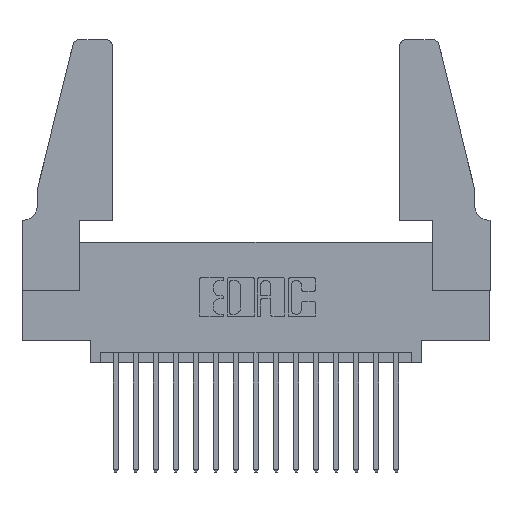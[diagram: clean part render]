
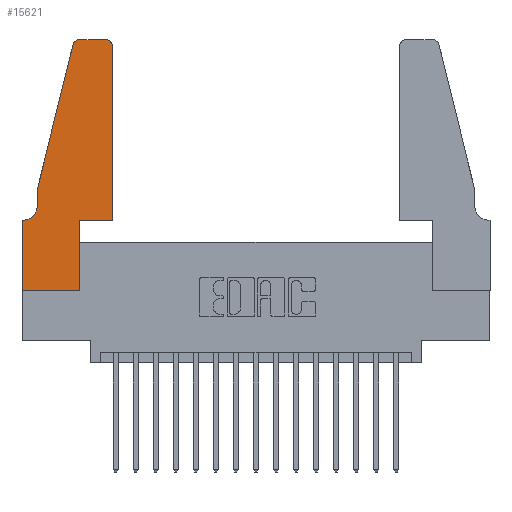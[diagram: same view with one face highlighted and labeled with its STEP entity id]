
A CAD part, top view. The second image highlights one B-rep face of the part: STEP entity #15621.
In plain terms, the highlighted planar face has unit normal (0, 0, 1).
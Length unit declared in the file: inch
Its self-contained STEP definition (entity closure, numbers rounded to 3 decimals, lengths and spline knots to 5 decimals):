
#3 = ORIENTED_EDGE ( 'NONE', *, *, #2744, .T. ) ;
#227 = EDGE_CURVE ( 'NONE', #11951, #13498, #530, .T. ) ;
#426 = CARTESIAN_POINT ( 'NONE',  ( 0.4505, 0.35, 0.37 ) ) ;
#530 = CIRCLE ( 'NONE', #17356, 0.03 ) ;
#564 = ORIENTED_EDGE ( 'NONE', *, *, #10258, .T. ) ;
#593 = CARTESIAN_POINT ( 'NONE',  ( 0.25487, 1.22718, 0.37 ) ) ;
#733 = CARTESIAN_POINT ( 'NONE',  ( 0.284, 1.22, 0.37 ) ) ;
#1566 = LINE ( 'NONE', #4669, #15255 ) ;
#1813 = LINE ( 'NONE', #7935, #13168 ) ;
#1875 = DIRECTION ( 'NONE',  ( 1., 0., 0. ) ) ;
#1921 = DIRECTION ( 'NONE',  ( 0., 0., 1. ) ) ;
#2294 = LINE ( 'NONE', #15361, #9162 ) ;
#2454 = DIRECTION ( 'NONE',  ( 0., 0., 1. ) ) ;
#2741 = ORIENTED_EDGE ( 'NONE', *, *, #15988, .T. ) ;
#2744 = EDGE_CURVE ( 'NONE', #3467, #5222, #1566, .T. ) ;
#2806 = CARTESIAN_POINT ( 'NONE',  ( 0.284, 1.25, 0.37 ) ) ;
#3303 = DIRECTION ( 'NONE',  ( 1., 0., 0. ) ) ;
#3320 = DIRECTION ( 'NONE',  ( 0., 0., 1. ) ) ;
#3467 = VERTEX_POINT ( 'NONE', #4648 ) ;
#3712 = EDGE_CURVE ( 'NONE', #12229, #3467, #1813, .T. ) ;
#4157 = DIRECTION ( 'NONE',  ( -0.239, -0.971, 0. ) ) ;
#4330 = VERTEX_POINT ( 'NONE', #14468 ) ;
#4384 = VECTOR ( 'NONE', #11359, 39.37008 ) ;
#4648 = CARTESIAN_POINT ( 'NONE',  ( 0., 0.35, 0.37 ) ) ;
#4669 = CARTESIAN_POINT ( 'NONE',  ( 0., 0., 0.37 ) ) ;
#4697 = EDGE_CURVE ( 'NONE', #10967, #6878, #7369, .T. ) ;
#5222 = VERTEX_POINT ( 'NONE', #8306 ) ;
#5450 = CARTESIAN_POINT ( 'NONE',  ( 0.0055, 0.42, 0.37 ) ) ;
#5584 = LINE ( 'NONE', #16413, #12421 ) ;
#5841 = DIRECTION ( 'NONE',  ( -1., 0., 0. ) ) ;
#5946 = EDGE_LOOP ( 'NONE', ( #8608, #14848, #11247, #11374, #2741, #7459, #3, #564, #16889, #15069, #6628, #9710 ) ) ;
#6025 = LINE ( 'NONE', #16396, #16035 ) ;
#6541 = CARTESIAN_POINT ( 'NONE',  ( 0.2865, 0., 0.37 ) ) ;
#6548 = AXIS2_PLACEMENT_3D ( 'NONE', #10142, #1921, #11499 ) ;
#6549 = VERTEX_POINT ( 'NONE', #14951 ) ;
#6628 = ORIENTED_EDGE ( 'NONE', *, *, #9845, .T. ) ;
#6826 = DIRECTION ( 'NONE',  ( -1., 0., 0. ) ) ;
#6878 = VERTEX_POINT ( 'NONE', #15640 ) ;
#7225 = CARTESIAN_POINT ( 'NONE',  ( 0.0755, 0.5, 0.37 ) ) ;
#7266 = EDGE_CURVE ( 'NONE', #13498, #10967, #5584, .T. ) ;
#7333 = FACE_OUTER_BOUND ( 'NONE', #5946, .T. ) ;
#7369 = LINE ( 'NONE', #10011, #4384 ) ;
#7459 = ORIENTED_EDGE ( 'NONE', *, *, #3712, .T. ) ;
#7738 = AXIS2_PLACEMENT_3D ( 'NONE', #11516, #3320, #12883 ) ;
#7935 = CARTESIAN_POINT ( 'NONE',  ( 0.0755, 0.35, 0.37 ) ) ;
#8149 = CIRCLE ( 'NONE', #7738, 0.03 ) ;
#8169 = VECTOR ( 'NONE', #15544, 39.37008 ) ;
#8306 = CARTESIAN_POINT ( 'NONE',  ( 0., 0., 0.37 ) ) ;
#8599 = LINE ( 'NONE', #14199, #8169 ) ;
#8608 = ORIENTED_EDGE ( 'NONE', *, *, #9064, .T. ) ;
#9064 = EDGE_CURVE ( 'NONE', #16120, #11951, #2294, .T. ) ;
#9162 = VECTOR ( 'NONE', #5841, 39.37008 ) ;
#9217 = AXIS2_PLACEMENT_3D ( 'NONE', #5450, #14985, #6826 ) ;
#9274 = LINE ( 'NONE', #15568, #12462 ) ;
#9710 = ORIENTED_EDGE ( 'NONE', *, *, #11013, .T. ) ;
#9845 = EDGE_CURVE ( 'NONE', #6549, #11124, #9274, .T. ) ;
#10011 = CARTESIAN_POINT ( 'NONE',  ( 0.0755, 0.5, 0.37 ) ) ;
#10142 = CARTESIAN_POINT ( 'NONE',  ( 0., 0.35, 0.37 ) ) ;
#10258 = EDGE_CURVE ( 'NONE', #5222, #17275, #6025, .T. ) ;
#10285 = LINE ( 'NONE', #426, #16645 ) ;
#10512 = EDGE_CURVE ( 'NONE', #17275, #4330, #8599, .T. ) ;
#10967 = VERTEX_POINT ( 'NONE', #7225 ) ;
#11013 = EDGE_CURVE ( 'NONE', #11124, #16120, #8149, .T. ) ;
#11124 = VERTEX_POINT ( 'NONE', #17143 ) ;
#11247 = ORIENTED_EDGE ( 'NONE', *, *, #7266, .T. ) ;
#11359 = DIRECTION ( 'NONE',  ( 0., -1., 0. ) ) ;
#11374 = ORIENTED_EDGE ( 'NONE', *, *, #4697, .T. ) ;
#11499 = DIRECTION ( 'NONE',  ( 1., 0., 0. ) ) ;
#11516 = CARTESIAN_POINT ( 'NONE',  ( 0.4205, 1.22, 0.37 ) ) ;
#11594 = CARTESIAN_POINT ( 'NONE',  ( 0.0055, 0.35, 0.37 ) ) ;
#11951 = VERTEX_POINT ( 'NONE', #2806 ) ;
#12229 = VERTEX_POINT ( 'NONE', #11594 ) ;
#12421 = VECTOR ( 'NONE', #4157, 39.37008 ) ;
#12462 = VECTOR ( 'NONE', #16941, 39.37008 ) ;
#12559 = CARTESIAN_POINT ( 'NONE',  ( 0.4205, 1.25, 0.37 ) ) ;
#12655 = CIRCLE ( 'NONE', #9217, 0.07 ) ;
#12883 = DIRECTION ( 'NONE',  ( 1., 0., 0. ) ) ;
#13168 = VECTOR ( 'NONE', #16006, 39.37008 ) ;
#13498 = VERTEX_POINT ( 'NONE', #593 ) ;
#14199 = CARTESIAN_POINT ( 'NONE',  ( 0.2865, 0.35, 0.37 ) ) ;
#14209 = DIRECTION ( 'NONE',  ( 0., -1., 0. ) ) ;
#14468 = CARTESIAN_POINT ( 'NONE',  ( 0.2865, 0.35, 0.37 ) ) ;
#14848 = ORIENTED_EDGE ( 'NONE', *, *, #227, .T. ) ;
#14951 = CARTESIAN_POINT ( 'NONE',  ( 0.4505, 0.35, 0.37 ) ) ;
#14985 = DIRECTION ( 'NONE',  ( 0., 0., -1. ) ) ;
#15035 = DIRECTION ( 'NONE',  ( 1., 0., 0. ) ) ;
#15069 = ORIENTED_EDGE ( 'NONE', *, *, #16872, .T. ) ;
#15255 = VECTOR ( 'NONE', #14209, 39.37008 ) ;
#15361 = CARTESIAN_POINT ( 'NONE',  ( 0.2605, 1.25, 0.37 ) ) ;
#15544 = DIRECTION ( 'NONE',  ( 0., 1., 0. ) ) ;
#15568 = CARTESIAN_POINT ( 'NONE',  ( 0.4505, 0.35, 0.37 ) ) ;
#15621 = ADVANCED_FACE ( 'NONE', ( #7333 ), #16887, .T. ) ;
#15640 = CARTESIAN_POINT ( 'NONE',  ( 0.0755, 0.42, 0.37 ) ) ;
#15988 = EDGE_CURVE ( 'NONE', #6878, #12229, #12655, .T. ) ;
#16006 = DIRECTION ( 'NONE',  ( -1., 0., 0. ) ) ;
#16035 = VECTOR ( 'NONE', #15035, 39.37008 ) ;
#16120 = VERTEX_POINT ( 'NONE', #12559 ) ;
#16396 = CARTESIAN_POINT ( 'NONE',  ( 0., 0., 0.37 ) ) ;
#16413 = CARTESIAN_POINT ( 'NONE',  ( 0.0755, 0.5, 0.37 ) ) ;
#16645 = VECTOR ( 'NONE', #1875, 39.37008 ) ;
#16872 = EDGE_CURVE ( 'NONE', #4330, #6549, #10285, .T. ) ;
#16887 = PLANE ( 'NONE',  #6548 ) ;
#16889 = ORIENTED_EDGE ( 'NONE', *, *, #10512, .T. ) ;
#16941 = DIRECTION ( 'NONE',  ( 0., 1., 0. ) ) ;
#17143 = CARTESIAN_POINT ( 'NONE',  ( 0.4505, 1.22, 0.37 ) ) ;
#17275 = VERTEX_POINT ( 'NONE', #6541 ) ;
#17356 = AXIS2_PLACEMENT_3D ( 'NONE', #733, #2454, #3303 ) ;
